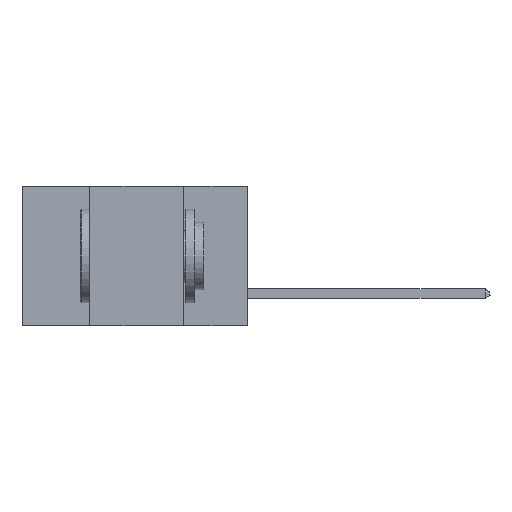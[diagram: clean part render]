
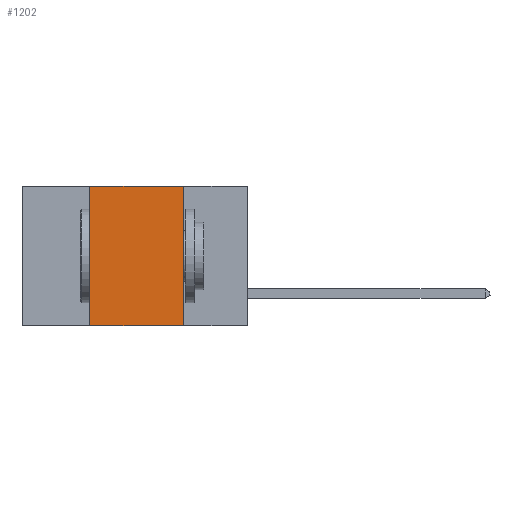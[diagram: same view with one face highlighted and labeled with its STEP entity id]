
A CAD part, left-side view. The second image highlights one B-rep face of the part: STEP entity #1202.
In plain terms, the highlighted planar face has unit normal (-1, 0, 0).
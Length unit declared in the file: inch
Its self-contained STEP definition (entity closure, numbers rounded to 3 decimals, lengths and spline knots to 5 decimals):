
#379 = CARTESIAN_POINT ( 'NONE',  ( 0., 0.6, 0. ) ) ;
#398 = VERTEX_POINT ( 'NONE', #10872 ) ;
#1101 = CARTESIAN_POINT ( 'NONE',  ( 0., 0.6, -0.37 ) ) ;
#1202 = ADVANCED_FACE ( 'NONE', ( #4536 ), #1810, .F. ) ;
#1221 = VERTEX_POINT ( 'NONE', #4715 ) ;
#1602 = VECTOR ( 'NONE', #11007, 39.37008 ) ;
#1633 = EDGE_CURVE ( 'NONE', #9193, #1221, #4140, .T. ) ;
#1810 = PLANE ( 'NONE',  #7779 ) ;
#1847 = DIRECTION ( 'NONE',  ( 0., 0., -1. ) ) ;
#1893 = CARTESIAN_POINT ( 'NONE',  ( 0., 0.6, 0. ) ) ;
#2400 = VECTOR ( 'NONE', #10560, 39.37008 ) ;
#2417 = CARTESIAN_POINT ( 'NONE',  ( 0., 0.42, 0. ) ) ;
#2472 = DIRECTION ( 'NONE',  ( 0., 0., -1. ) ) ;
#2866 = LINE ( 'NONE', #379, #4208 ) ;
#2929 = ORIENTED_EDGE ( 'NONE', *, *, #4459, .F. ) ;
#3056 = ORIENTED_EDGE ( 'NONE', *, *, #9514, .T. ) ;
#3369 = VERTEX_POINT ( 'NONE', #8073 ) ;
#4058 = EDGE_LOOP ( 'NONE', ( #4213, #2929, #5597, #3056 ) ) ;
#4140 = LINE ( 'NONE', #2417, #1602 ) ;
#4208 = VECTOR ( 'NONE', #4255, 39.37008 ) ;
#4213 = ORIENTED_EDGE ( 'NONE', *, *, #7226, .F. ) ;
#4255 = DIRECTION ( 'NONE',  ( 0., -1., 0. ) ) ;
#4459 = EDGE_CURVE ( 'NONE', #1221, #398, #2866, .T. ) ;
#4536 = FACE_OUTER_BOUND ( 'NONE', #4058, .T. ) ;
#4715 = CARTESIAN_POINT ( 'NONE',  ( 0., 0.42, 0. ) ) ;
#5276 = CARTESIAN_POINT ( 'NONE',  ( 0., 0.42, -0.37 ) ) ;
#5597 = ORIENTED_EDGE ( 'NONE', *, *, #1633, .F. ) ;
#7226 = EDGE_CURVE ( 'NONE', #398, #3369, #8332, .T. ) ;
#7779 = AXIS2_PLACEMENT_3D ( 'NONE', #1893, #10433, #1847 ) ;
#8072 = LINE ( 'NONE', #1101, #2400 ) ;
#8073 = CARTESIAN_POINT ( 'NONE',  ( 0., 0.17, -0.37 ) ) ;
#8332 = LINE ( 'NONE', #10144, #9105 ) ;
#9105 = VECTOR ( 'NONE', #2472, 39.37008 ) ;
#9193 = VERTEX_POINT ( 'NONE', #5276 ) ;
#9514 = EDGE_CURVE ( 'NONE', #9193, #3369, #8072, .T. ) ;
#10144 = CARTESIAN_POINT ( 'NONE',  ( 0., 0.17, 0. ) ) ;
#10433 = DIRECTION ( 'NONE',  ( 1., 0., 0. ) ) ;
#10560 = DIRECTION ( 'NONE',  ( 0., -1., 0. ) ) ;
#10872 = CARTESIAN_POINT ( 'NONE',  ( 0., 0.17, 0. ) ) ;
#11007 = DIRECTION ( 'NONE',  ( 0., 0., 1. ) ) ;
